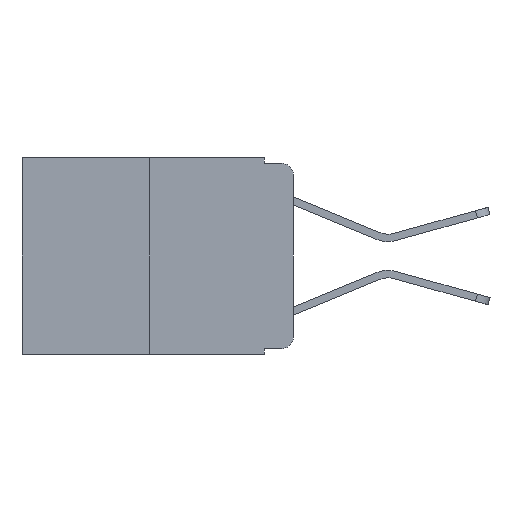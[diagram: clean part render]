
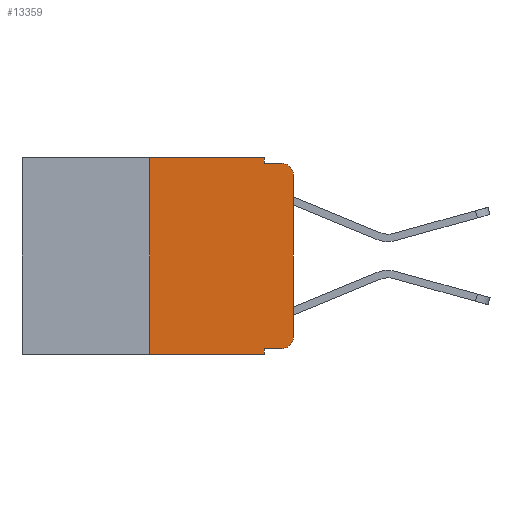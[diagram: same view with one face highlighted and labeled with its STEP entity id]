
A CAD part, left-side view. The second image highlights one B-rep face of the part: STEP entity #13359.
In plain terms, the highlighted planar face has unit normal (-1, 0, 0).
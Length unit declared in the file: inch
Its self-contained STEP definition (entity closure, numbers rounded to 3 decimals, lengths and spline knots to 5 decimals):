
#389 = VERTEX_POINT ( 'NONE', #11096 ) ;
#1170 = DIRECTION ( 'NONE',  ( 0., -1., 0. ) ) ;
#1191 = VECTOR ( 'NONE', #1170, 39.37008 ) ;
#1495 = AXIS2_PLACEMENT_3D ( 'NONE', #13028, #15226, #2283 ) ;
#1578 = EDGE_CURVE ( 'NONE', #13276, #11560, #3070, .T. ) ;
#1592 = DIRECTION ( 'NONE',  ( 0., 0., -1. ) ) ;
#2283 = DIRECTION ( 'NONE',  ( 0., 0., -1. ) ) ;
#2444 = VECTOR ( 'NONE', #6180, 39.37008 ) ;
#2503 = CARTESIAN_POINT ( 'NONE',  ( 0., 0.02, -0.03 ) ) ;
#2932 = DIRECTION ( 'NONE',  ( 0., 0., 1. ) ) ;
#2933 = CIRCLE ( 'NONE', #1495, 0.02 ) ;
#3070 = LINE ( 'NONE', #13229, #13739 ) ;
#3266 = DIRECTION ( 'NONE',  ( 0., 0., -1. ) ) ;
#3582 = ORIENTED_EDGE ( 'NONE', *, *, #14648, .T. ) ;
#3703 = EDGE_CURVE ( 'NONE', #13276, #10966, #13844, .T. ) ;
#3724 = LINE ( 'NONE', #14046, #5594 ) ;
#3957 = EDGE_CURVE ( 'NONE', #389, #7790, #3724, .T. ) ;
#4086 = CARTESIAN_POINT ( 'NONE',  ( 0., 0.25, -0.343 ) ) ;
#4733 = ORIENTED_EDGE ( 'NONE', *, *, #5638, .F. ) ;
#4844 = CARTESIAN_POINT ( 'NONE',  ( 0., 0.473, 0. ) ) ;
#5113 = CARTESIAN_POINT ( 'NONE',  ( 0., 0.051, -0.01 ) ) ;
#5127 = PLANE ( 'NONE',  #14628 ) ;
#5293 = DIRECTION ( 'NONE',  ( 0., 0., -1. ) ) ;
#5412 = CARTESIAN_POINT ( 'NONE',  ( 0., 0., -0.03 ) ) ;
#5594 = VECTOR ( 'NONE', #3266, 39.37008 ) ;
#5638 = EDGE_CURVE ( 'NONE', #11972, #389, #10229, .T. ) ;
#6180 = DIRECTION ( 'NONE',  ( 0., -1., 0. ) ) ;
#6345 = ORIENTED_EDGE ( 'NONE', *, *, #10033, .F. ) ;
#6397 = ORIENTED_EDGE ( 'NONE', *, *, #8494, .T. ) ;
#6459 = LINE ( 'NONE', #9380, #12526 ) ;
#6833 = ORIENTED_EDGE ( 'NONE', *, *, #8490, .F. ) ;
#7203 = LINE ( 'NONE', #5113, #14904 ) ;
#7346 = VECTOR ( 'NONE', #2932, 39.37008 ) ;
#7408 = CARTESIAN_POINT ( 'NONE',  ( 0., 0.02, -0.333 ) ) ;
#7790 = VERTEX_POINT ( 'NONE', #14464 ) ;
#7967 = CARTESIAN_POINT ( 'NONE',  ( 0., 0., -0.313 ) ) ;
#8403 = ORIENTED_EDGE ( 'NONE', *, *, #3703, .T. ) ;
#8470 = VERTEX_POINT ( 'NONE', #12815 ) ;
#8490 = EDGE_CURVE ( 'NONE', #7790, #8470, #7203, .T. ) ;
#8494 = EDGE_CURVE ( 'NONE', #13328, #11560, #6459, .T. ) ;
#8552 = EDGE_CURVE ( 'NONE', #9863, #8470, #14552, .T. ) ;
#8874 = AXIS2_PLACEMENT_3D ( 'NONE', #2503, #12113, #10765 ) ;
#9282 = DIRECTION ( 'NONE',  ( 0., -1., 0. ) ) ;
#9380 = CARTESIAN_POINT ( 'NONE',  ( 0., 0.473, -0.343 ) ) ;
#9389 = DIRECTION ( 'NONE',  ( 0., -1., 0. ) ) ;
#9863 = VERTEX_POINT ( 'NONE', #5412 ) ;
#9894 = CARTESIAN_POINT ( 'NONE',  ( 0., 0.051, -0.333 ) ) ;
#9938 = ORIENTED_EDGE ( 'NONE', *, *, #3957, .F. ) ;
#10033 = EDGE_CURVE ( 'NONE', #13328, #11972, #14335, .T. ) ;
#10203 = EDGE_CURVE ( 'NONE', #10966, #14217, #2933, .T. ) ;
#10229 = LINE ( 'NONE', #4844, #1191 ) ;
#10318 = ORIENTED_EDGE ( 'NONE', *, *, #1578, .F. ) ;
#10419 = DIRECTION ( 'NONE',  ( 0., 0., 1. ) ) ;
#10687 = VECTOR ( 'NONE', #10419, 39.37008 ) ;
#10708 = FACE_OUTER_BOUND ( 'NONE', #11846, .T. ) ;
#10765 = DIRECTION ( 'NONE',  ( 0., 0., -1. ) ) ;
#10966 = VERTEX_POINT ( 'NONE', #7408 ) ;
#11096 = CARTESIAN_POINT ( 'NONE',  ( 0., 0.051, 0. ) ) ;
#11145 = CARTESIAN_POINT ( 'NONE',  ( 0., 0.473, 0. ) ) ;
#11560 = VERTEX_POINT ( 'NONE', #14165 ) ;
#11842 = CARTESIAN_POINT ( 'NONE',  ( 0., 0.25, 0. ) ) ;
#11846 = EDGE_LOOP ( 'NONE', ( #3582, #14262, #6833, #9938, #4733, #6345, #6397, #10318, #8403, #13394 ) ) ;
#11972 = VERTEX_POINT ( 'NONE', #11842 ) ;
#12020 = CARTESIAN_POINT ( 'NONE',  ( 0., 0.051, -0.333 ) ) ;
#12113 = DIRECTION ( 'NONE',  ( -1., 0., 0. ) ) ;
#12432 = CARTESIAN_POINT ( 'NONE',  ( 0., 0., 0. ) ) ;
#12526 = VECTOR ( 'NONE', #9389, 39.37008 ) ;
#12815 = CARTESIAN_POINT ( 'NONE',  ( 0., 0.02, -0.01 ) ) ;
#13028 = CARTESIAN_POINT ( 'NONE',  ( 0., 0.02, -0.313 ) ) ;
#13229 = CARTESIAN_POINT ( 'NONE',  ( 0., 0.051, 0. ) ) ;
#13276 = VERTEX_POINT ( 'NONE', #9894 ) ;
#13328 = VERTEX_POINT ( 'NONE', #4086 ) ;
#13359 = ADVANCED_FACE ( 'NONE', ( #10708 ), #5127, .F. ) ;
#13394 = ORIENTED_EDGE ( 'NONE', *, *, #10203, .T. ) ;
#13739 = VECTOR ( 'NONE', #1592, 39.37008 ) ;
#13844 = LINE ( 'NONE', #12020, #2444 ) ;
#14046 = CARTESIAN_POINT ( 'NONE',  ( 0., 0.051, 0. ) ) ;
#14165 = CARTESIAN_POINT ( 'NONE',  ( 0., 0.051, -0.343 ) ) ;
#14217 = VERTEX_POINT ( 'NONE', #7967 ) ;
#14262 = ORIENTED_EDGE ( 'NONE', *, *, #8552, .T. ) ;
#14335 = LINE ( 'NONE', #15074, #10687 ) ;
#14464 = CARTESIAN_POINT ( 'NONE',  ( 0., 0.051, -0.01 ) ) ;
#14523 = DIRECTION ( 'NONE',  ( 1., 0., 0. ) ) ;
#14552 = CIRCLE ( 'NONE', #8874, 0.02 ) ;
#14628 = AXIS2_PLACEMENT_3D ( 'NONE', #11145, #14523, #5293 ) ;
#14648 = EDGE_CURVE ( 'NONE', #14217, #9863, #14690, .T. ) ;
#14690 = LINE ( 'NONE', #12432, #7346 ) ;
#14904 = VECTOR ( 'NONE', #9282, 39.37008 ) ;
#15074 = CARTESIAN_POINT ( 'NONE',  ( 0., 0.25, 0. ) ) ;
#15226 = DIRECTION ( 'NONE',  ( -1., 0., 0. ) ) ;
